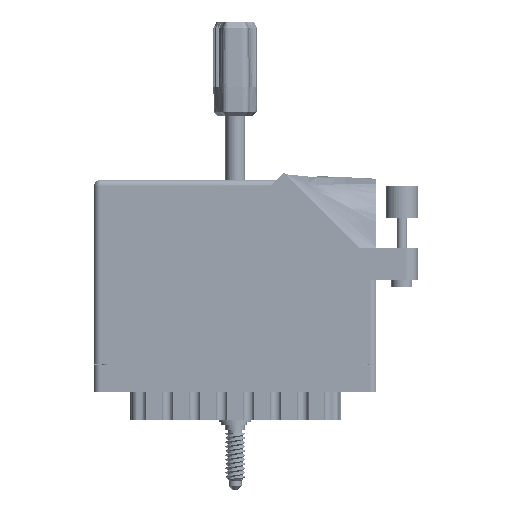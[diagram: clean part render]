
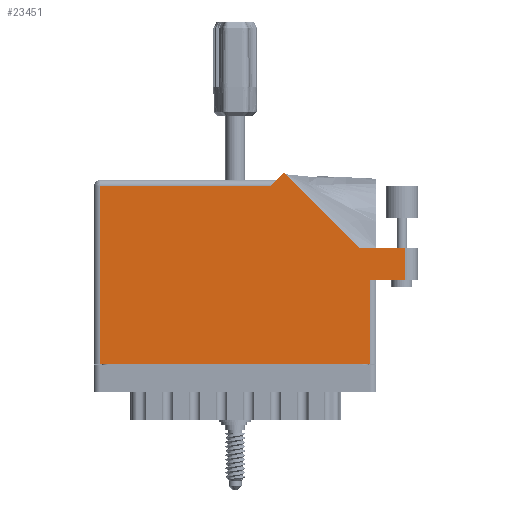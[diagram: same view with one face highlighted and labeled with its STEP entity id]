
A CAD part, front view. The second image highlights one B-rep face of the part: STEP entity #23451.
In plain terms, the highlighted face is planar.
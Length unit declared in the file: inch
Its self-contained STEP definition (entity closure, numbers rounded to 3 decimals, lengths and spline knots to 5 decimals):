
#1105 = DIRECTION ( 'NONE',  ( 0., 1., 0. ) ) ;
#2022 = CARTESIAN_POINT ( 'NONE',  ( 2.656, 0.815, 0. ) ) ;
#2285 = VERTEX_POINT ( 'NONE', #83341 ) ;
#3573 = LINE ( 'NONE', #60009, #13224 ) ;
#4482 = VERTEX_POINT ( 'NONE', #23571 ) ;
#4989 = EDGE_CURVE ( 'NONE', #74198, #25668, #11428, .T. ) ;
#5144 = VERTEX_POINT ( 'NONE', #75186 ) ;
#5932 = CARTESIAN_POINT ( 'NONE',  ( 2.718, 0.815, 0. ) ) ;
#7032 = DIRECTION ( 'NONE',  ( -0.707, 0.707, 0. ) ) ;
#7496 = AXIS2_PLACEMENT_3D ( 'NONE', #41603, #48888, #48279 ) ;
#8687 = VECTOR ( 'NONE', #26767, 39.37008 ) ;
#10711 = VECTOR ( 'NONE', #7032, 39.37008 ) ;
#11428 = LINE ( 'NONE', #61702, #82728 ) ;
#13093 = CARTESIAN_POINT ( 'NONE',  ( 0., 1.713, 0. ) ) ;
#13224 = VECTOR ( 'NONE', #21261, 39.37008 ) ;
#14391 = CARTESIAN_POINT ( 'NONE',  ( 2.993, 1.122, 0. ) ) ;
#14446 = DIRECTION ( 'NONE',  ( 0., 1., 0. ) ) ;
#17183 = EDGE_CURVE ( 'NONE', #25668, #28961, #89368, .T. ) ;
#20525 = PLANE ( 'NONE',  #7496 ) ;
#21261 = DIRECTION ( 'NONE',  ( 1., 0., 0. ) ) ;
#22378 = VERTEX_POINT ( 'NONE', #84727 ) ;
#23451 = ADVANCED_FACE ( 'NONE', ( #83271 ), #20525, .F. ) ;
#23571 = CARTESIAN_POINT ( 'NONE',  ( 2.656, 0., 0. ) ) ;
#23722 = VECTOR ( 'NONE', #1105, 39.37008 ) ;
#25668 = VERTEX_POINT ( 'NONE', #32219 ) ;
#26767 = DIRECTION ( 'NONE',  ( 1., 0., 0. ) ) ;
#26961 = LINE ( 'NONE', #65472, #52875 ) ;
#27785 = CARTESIAN_POINT ( 'NONE',  ( 0.062, 1.713, 0. ) ) ;
#28961 = VERTEX_POINT ( 'NONE', #27785 ) ;
#30257 = LINE ( 'NONE', #14391, #83187 ) ;
#30495 = CARTESIAN_POINT ( 'NONE',  ( 0.062, 0., 0. ) ) ;
#32219 = CARTESIAN_POINT ( 'NONE',  ( 1.696, 1.713, 0. ) ) ;
#37731 = LINE ( 'NONE', #2022, #23722 ) ;
#38569 = EDGE_CURVE ( 'NONE', #4482, #70098, #37731, .T. ) ;
#38831 = CARTESIAN_POINT ( 'NONE',  ( 1.82871, 1.84571, 0. ) ) ;
#41603 = CARTESIAN_POINT ( 'NONE',  ( 0., 1.775, 0. ) ) ;
#44176 = VECTOR ( 'NONE', #52152, 39.37008 ) ;
#45266 = EDGE_LOOP ( 'NONE', ( #66957, #54648, #70363, #87812, #70900, #69047, #79891, #57081, #62446 ) ) ;
#46304 = EDGE_CURVE ( 'NONE', #5144, #2285, #30257, .T. ) ;
#46468 = EDGE_CURVE ( 'NONE', #2285, #22378, #47460, .T. ) ;
#47460 = LINE ( 'NONE', #51569, #44176 ) ;
#48279 = DIRECTION ( 'NONE',  ( -1., 0., 0. ) ) ;
#48888 = DIRECTION ( 'NONE',  ( 0., 0., -1. ) ) ;
#51569 = CARTESIAN_POINT ( 'NONE',  ( 3.118, 1.122, 0. ) ) ;
#51935 = VERTEX_POINT ( 'NONE', #30495 ) ;
#52152 = DIRECTION ( 'NONE',  ( -1., 0., 0. ) ) ;
#52875 = VECTOR ( 'NONE', #58521, 39.37008 ) ;
#54648 = ORIENTED_EDGE ( 'NONE', *, *, #46304, .T. ) ;
#54726 = DIRECTION ( 'NONE',  ( -1., 0., 0. ) ) ;
#57081 = ORIENTED_EDGE ( 'NONE', *, *, #70674, .T. ) ;
#58521 = DIRECTION ( 'NONE',  ( 0., -1., 0. ) ) ;
#58983 = EDGE_CURVE ( 'NONE', #22378, #74198, #67937, .T. ) ;
#60009 = CARTESIAN_POINT ( 'NONE',  ( 0., 0., 0. ) ) ;
#61303 = CARTESIAN_POINT ( 'NONE',  ( 2.656, 0.815, 0. ) ) ;
#61702 = CARTESIAN_POINT ( 'NONE',  ( 1.758, 1.775, 0. ) ) ;
#62446 = ORIENTED_EDGE ( 'NONE', *, *, #38569, .T. ) ;
#65472 = CARTESIAN_POINT ( 'NONE',  ( 0.062, 0., 0. ) ) ;
#66630 = VECTOR ( 'NONE', #54726, 39.37008 ) ;
#66957 = ORIENTED_EDGE ( 'NONE', *, *, #88317, .T. ) ;
#67937 = LINE ( 'NONE', #83715, #10711 ) ;
#69047 = ORIENTED_EDGE ( 'NONE', *, *, #17183, .T. ) ;
#70098 = VERTEX_POINT ( 'NONE', #61303 ) ;
#70363 = ORIENTED_EDGE ( 'NONE', *, *, #46468, .T. ) ;
#70674 = EDGE_CURVE ( 'NONE', #51935, #4482, #3573, .T. ) ;
#70900 = ORIENTED_EDGE ( 'NONE', *, *, #4989, .T. ) ;
#74198 = VERTEX_POINT ( 'NONE', #38831 ) ;
#75186 = CARTESIAN_POINT ( 'NONE',  ( 2.993, 0.815, 0. ) ) ;
#79891 = ORIENTED_EDGE ( 'NONE', *, *, #89229, .T. ) ;
#82554 = DIRECTION ( 'NONE',  ( -0.707, -0.707, 0. ) ) ;
#82728 = VECTOR ( 'NONE', #82554, 39.37008 ) ;
#83187 = VECTOR ( 'NONE', #14446, 39.37008 ) ;
#83271 = FACE_OUTER_BOUND ( 'NONE', #45266, .T. ) ;
#83341 = CARTESIAN_POINT ( 'NONE',  ( 2.993, 1.122, 0. ) ) ;
#83715 = CARTESIAN_POINT ( 'NONE',  ( 2.55242, 1.122, 0. ) ) ;
#84727 = CARTESIAN_POINT ( 'NONE',  ( 2.55242, 1.122, 0. ) ) ;
#87630 = LINE ( 'NONE', #5932, #8687 ) ;
#87812 = ORIENTED_EDGE ( 'NONE', *, *, #58983, .T. ) ;
#88317 = EDGE_CURVE ( 'NONE', #70098, #5144, #87630, .T. ) ;
#89229 = EDGE_CURVE ( 'NONE', #28961, #51935, #26961, .T. ) ;
#89368 = LINE ( 'NONE', #13093, #66630 ) ;
